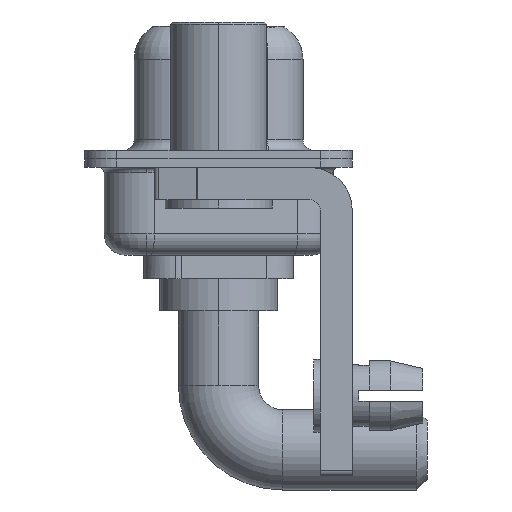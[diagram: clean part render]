
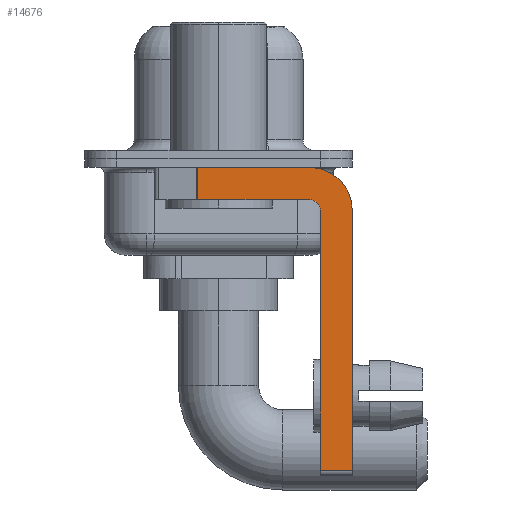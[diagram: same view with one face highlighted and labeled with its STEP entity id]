
A CAD part, left-side view. The second image highlights one B-rep face of the part: STEP entity #14676.
In plain terms, the highlighted planar face has unit normal (-1, 0, 0).
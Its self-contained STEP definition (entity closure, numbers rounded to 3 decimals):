
#9 = CARTESIAN_POINT ( 'NONE',  ( -2.9, -4.25, -14.55 ) ) ;
#45 = DIRECTION ( 'NONE',  ( 0., 0., -1. ) ) ;
#139 = DIRECTION ( 'NONE',  ( 0., 0., 1. ) ) ;
#159 = DIRECTION ( 'NONE',  ( 0., 0., -1. ) ) ;
#311 = DIRECTION ( 'NONE',  ( -1., 0., 0. ) ) ;
#409 = CARTESIAN_POINT ( 'NONE',  ( -2.9, -4.25, -2.4 ) ) ;
#414 = AXIS2_PLACEMENT_3D ( 'NONE', #9423, #311, #139 ) ;
#791 = ORIENTED_EDGE ( 'NONE', *, *, #2663, .F. ) ;
#867 = EDGE_CURVE ( 'NONE', #14470, #5979, #14486, .T. ) ;
#982 = LINE ( 'NONE', #16614, #11711 ) ;
#1169 = LINE ( 'NONE', #4088, #16717 ) ;
#1682 = DIRECTION ( 'NONE',  ( 1., 0., 0. ) ) ;
#1689 = VERTEX_POINT ( 'NONE', #7332 ) ;
#2125 = CARTESIAN_POINT ( 'NONE',  ( -2.9, -6.25, -2.4 ) ) ;
#2325 = VECTOR ( 'NONE', #9113, 1000. ) ;
#2663 = EDGE_CURVE ( 'NONE', #12365, #14470, #14839, .T. ) ;
#2888 = LINE ( 'NONE', #9, #2325 ) ;
#3328 = CARTESIAN_POINT ( 'NONE',  ( -2.9, -4.75, -14.55 ) ) ;
#3909 = CARTESIAN_POINT ( 'NONE',  ( -2.9, -4.25, -0.4 ) ) ;
#3998 = EDGE_CURVE ( 'NONE', #15593, #1689, #1169, .T. ) ;
#4088 = CARTESIAN_POINT ( 'NONE',  ( -2.9, 0.978, -1.9 ) ) ;
#4293 = DIRECTION ( 'NONE',  ( 0., 1., 0. ) ) ;
#4365 = ORIENTED_EDGE ( 'NONE', *, *, #13019, .F. ) ;
#4877 = VECTOR ( 'NONE', #159, 1000. ) ;
#4925 = DIRECTION ( 'NONE',  ( 0., -1., 0. ) ) ;
#5349 = CARTESIAN_POINT ( 'NONE',  ( -2.9, -6.25, -14.55 ) ) ;
#5536 = EDGE_CURVE ( 'NONE', #11786, #5979, #2888, .T. ) ;
#5979 = VERTEX_POINT ( 'NONE', #5349 ) ;
#6230 = ORIENTED_EDGE ( 'NONE', *, *, #11613, .F. ) ;
#6507 = ORIENTED_EDGE ( 'NONE', *, *, #867, .F. ) ;
#6733 = FACE_OUTER_BOUND ( 'NONE', #12077, .T. ) ;
#7287 = CARTESIAN_POINT ( 'NONE',  ( -2.9, 0.978, -0.4 ) ) ;
#7332 = CARTESIAN_POINT ( 'NONE',  ( -2.9, 0.978, -1.9 ) ) ;
#7839 = DIRECTION ( 'NONE',  ( 0., 0., -1. ) ) ;
#7964 = ORIENTED_EDGE ( 'NONE', *, *, #15253, .F. ) ;
#7995 = VECTOR ( 'NONE', #11262, 1000. ) ;
#8859 = CIRCLE ( 'NONE', #414, 0.5 ) ;
#9113 = DIRECTION ( 'NONE',  ( 0., -1., 0. ) ) ;
#9200 = PLANE ( 'NONE',  #16207 ) ;
#9423 = CARTESIAN_POINT ( 'NONE',  ( -2.9, -4.25, -2.4 ) ) ;
#10295 = ORIENTED_EDGE ( 'NONE', *, *, #13985, .F. ) ;
#10433 = CARTESIAN_POINT ( 'NONE',  ( -2.9, -4.25, -2.4 ) ) ;
#11262 = DIRECTION ( 'NONE',  ( 0., 0., 1. ) ) ;
#11613 = EDGE_CURVE ( 'NONE', #12371, #1689, #16060, .T. ) ;
#11711 = VECTOR ( 'NONE', #4925, 1000. ) ;
#11786 = VERTEX_POINT ( 'NONE', #3328 ) ;
#12077 = EDGE_LOOP ( 'NONE', ( #4365, #16070, #6230, #7964, #10295, #16599, #6507, #791 ) ) ;
#12365 = VERTEX_POINT ( 'NONE', #3909 ) ;
#12371 = VERTEX_POINT ( 'NONE', #12698 ) ;
#12551 = CARTESIAN_POINT ( 'NONE',  ( -2.9, -4.75, -14.8 ) ) ;
#12698 = CARTESIAN_POINT ( 'NONE',  ( -2.9, -4.25, -1.9 ) ) ;
#12997 = VERTEX_POINT ( 'NONE', #14290 ) ;
#13019 = EDGE_CURVE ( 'NONE', #15593, #12365, #982, .T. ) ;
#13613 = VECTOR ( 'NONE', #4293, 1000. ) ;
#13832 = LINE ( 'NONE', #12551, #7995 ) ;
#13985 = EDGE_CURVE ( 'NONE', #11786, #12997, #13832, .T. ) ;
#14290 = CARTESIAN_POINT ( 'NONE',  ( -2.9, -4.75, -2.4 ) ) ;
#14470 = VERTEX_POINT ( 'NONE', #2125 ) ;
#14486 = LINE ( 'NONE', #15601, #4877 ) ;
#14676 = ADVANCED_FACE ( 'NONE', ( #6733 ), #9200, .F. ) ;
#14839 = CIRCLE ( 'NONE', #15402, 2. ) ;
#15253 = EDGE_CURVE ( 'NONE', #12997, #12371, #8859, .T. ) ;
#15393 = DIRECTION ( 'NONE',  ( 1., 0., 0. ) ) ;
#15402 = AXIS2_PLACEMENT_3D ( 'NONE', #10433, #15393, #45 ) ;
#15593 = VERTEX_POINT ( 'NONE', #7287 ) ;
#15601 = CARTESIAN_POINT ( 'NONE',  ( -2.9, -6.25, -2.4 ) ) ;
#15773 = DIRECTION ( 'NONE',  ( 0., 0., -1. ) ) ;
#15971 = CARTESIAN_POINT ( 'NONE',  ( -2.9, -4.25, -1.9 ) ) ;
#16060 = LINE ( 'NONE', #15971, #13613 ) ;
#16070 = ORIENTED_EDGE ( 'NONE', *, *, #3998, .T. ) ;
#16207 = AXIS2_PLACEMENT_3D ( 'NONE', #409, #1682, #15773 ) ;
#16599 = ORIENTED_EDGE ( 'NONE', *, *, #5536, .T. ) ;
#16614 = CARTESIAN_POINT ( 'NONE',  ( -2.9, 3., -0.4 ) ) ;
#16717 = VECTOR ( 'NONE', #7839, 1000. ) ;
